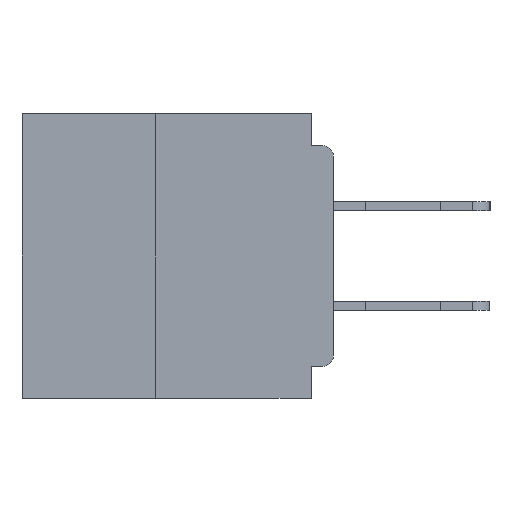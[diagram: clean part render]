
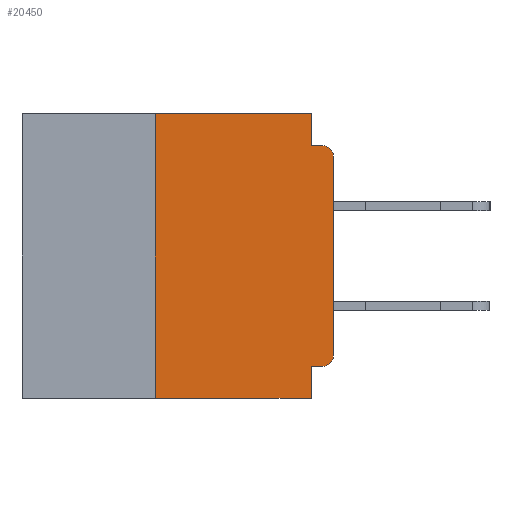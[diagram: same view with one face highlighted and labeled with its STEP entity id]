
A CAD part, left-side view. The second image highlights one B-rep face of the part: STEP entity #20450.
In plain terms, the highlighted planar face has unit normal (-1, 0, 0).
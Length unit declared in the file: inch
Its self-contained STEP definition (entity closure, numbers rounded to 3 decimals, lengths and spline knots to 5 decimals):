
#257 = EDGE_CURVE ( 'NONE', #21240, #16895, #29315, .T. ) ;
#332 = DIRECTION ( 'NONE',  ( -1., 0., 0. ) ) ;
#970 = CARTESIAN_POINT ( 'NONE',  ( 0., 0.015, -0.045 ) ) ;
#2657 = CARTESIAN_POINT ( 'NONE',  ( 0., 0.031, -0.045 ) ) ;
#2913 = LINE ( 'NONE', #9096, #38923 ) ;
#4142 = CARTESIAN_POINT ( 'NONE',  ( 0., 0., -0.34 ) ) ;
#5055 = VECTOR ( 'NONE', #23852, 39.37008 ) ;
#5239 = VERTEX_POINT ( 'NONE', #36201 ) ;
#6956 = VERTEX_POINT ( 'NONE', #32153 ) ;
#8666 = VERTEX_POINT ( 'NONE', #28612 ) ;
#9096 = CARTESIAN_POINT ( 'NONE',  ( 0., 0., 0. ) ) ;
#9192 = LINE ( 'NONE', #13168, #24970 ) ;
#9585 = VECTOR ( 'NONE', #23158, 39.37008 ) ;
#10369 = ORIENTED_EDGE ( 'NONE', *, *, #34134, .T. ) ;
#10654 = DIRECTION ( 'NONE',  ( 0., 0., -1. ) ) ;
#10909 = EDGE_CURVE ( 'NONE', #5239, #39149, #43585, .T. ) ;
#11137 = ORIENTED_EDGE ( 'NONE', *, *, #34809, .T. ) ;
#11266 = VERTEX_POINT ( 'NONE', #11587 ) ;
#11587 = CARTESIAN_POINT ( 'NONE',  ( 0., 0.25, -0.4 ) ) ;
#12026 = AXIS2_PLACEMENT_3D ( 'NONE', #34655, #13116, #38203 ) ;
#13116 = DIRECTION ( 'NONE',  ( -1., 0., 0. ) ) ;
#13168 = CARTESIAN_POINT ( 'NONE',  ( 0., 0.437, -0.4 ) ) ;
#13255 = ORIENTED_EDGE ( 'NONE', *, *, #10909, .F. ) ;
#13283 = ORIENTED_EDGE ( 'NONE', *, *, #257, .F. ) ;
#13321 = EDGE_CURVE ( 'NONE', #11266, #39149, #9192, .T. ) ;
#14574 = EDGE_CURVE ( 'NONE', #16895, #30800, #29369, .T. ) ;
#15464 = PLANE ( 'NONE',  #26780 ) ;
#16793 = EDGE_CURVE ( 'NONE', #6956, #5239, #33820, .T. ) ;
#16895 = VERTEX_POINT ( 'NONE', #2657 ) ;
#18525 = DIRECTION ( 'NONE',  ( 0., -1., 0. ) ) ;
#18948 = CARTESIAN_POINT ( 'NONE',  ( 0., 0.031, -0.4 ) ) ;
#19184 = LINE ( 'NONE', #37280, #9585 ) ;
#20450 = ADVANCED_FACE ( 'NONE', ( #27389 ), #15464, .F. ) ;
#20467 = DIRECTION ( 'NONE',  ( 0., 0., -1. ) ) ;
#21240 = VERTEX_POINT ( 'NONE', #41824 ) ;
#22002 = CARTESIAN_POINT ( 'NONE',  ( 0., 0.015, -0.06 ) ) ;
#22453 = DIRECTION ( 'NONE',  ( 0., 0., 1. ) ) ;
#22488 = CIRCLE ( 'NONE', #12026, 0.015 ) ;
#22690 = DIRECTION ( 'NONE',  ( 0., 0., -1. ) ) ;
#23158 = DIRECTION ( 'NONE',  ( 0., 0., 1. ) ) ;
#23670 = EDGE_CURVE ( 'NONE', #6956, #42886, #22488, .T. ) ;
#23852 = DIRECTION ( 'NONE',  ( 0., 1., 0. ) ) ;
#24042 = DIRECTION ( 'NONE',  ( 0., -1., 0. ) ) ;
#24398 = ORIENTED_EDGE ( 'NONE', *, *, #16793, .F. ) ;
#24970 = VECTOR ( 'NONE', #24042, 39.37008 ) ;
#24983 = ORIENTED_EDGE ( 'NONE', *, *, #13321, .T. ) ;
#25650 = DIRECTION ( 'NONE',  ( 0., 0., -1. ) ) ;
#26780 = AXIS2_PLACEMENT_3D ( 'NONE', #40483, #44033, #22690 ) ;
#27389 = FACE_OUTER_BOUND ( 'NONE', #42995, .T. ) ;
#28597 = ORIENTED_EDGE ( 'NONE', *, *, #14574, .F. ) ;
#28612 = CARTESIAN_POINT ( 'NONE',  ( 0., 0., -0.06 ) ) ;
#29315 = LINE ( 'NONE', #43407, #37644 ) ;
#29369 = LINE ( 'NONE', #38201, #44864 ) ;
#30227 = EDGE_CURVE ( 'NONE', #11266, #41132, #19184, .T. ) ;
#30800 = VERTEX_POINT ( 'NONE', #970 ) ;
#31580 = VECTOR ( 'NONE', #18525, 39.37008 ) ;
#32153 = CARTESIAN_POINT ( 'NONE',  ( 0., 0.015, -0.355 ) ) ;
#33820 = LINE ( 'NONE', #41613, #5055 ) ;
#34134 = EDGE_CURVE ( 'NONE', #42886, #8666, #2913, .T. ) ;
#34188 = VECTOR ( 'NONE', #20467, 39.37008 ) ;
#34655 = CARTESIAN_POINT ( 'NONE',  ( 0., 0.015, -0.34 ) ) ;
#34809 = EDGE_CURVE ( 'NONE', #8666, #30800, #37214, .T. ) ;
#36201 = CARTESIAN_POINT ( 'NONE',  ( 0., 0.031, -0.355 ) ) ;
#37214 = CIRCLE ( 'NONE', #44979, 0.015 ) ;
#37280 = CARTESIAN_POINT ( 'NONE',  ( 0., 0.25, -0.4 ) ) ;
#37644 = VECTOR ( 'NONE', #10654, 39.37008 ) ;
#38110 = ORIENTED_EDGE ( 'NONE', *, *, #44725, .F. ) ;
#38201 = CARTESIAN_POINT ( 'NONE',  ( 0., 0., -0.045 ) ) ;
#38203 = DIRECTION ( 'NONE',  ( 0., 0., -1. ) ) ;
#38281 = CARTESIAN_POINT ( 'NONE',  ( 0., 0.25, 0. ) ) ;
#38361 = DIRECTION ( 'NONE',  ( 0., -1., 0. ) ) ;
#38534 = ORIENTED_EDGE ( 'NONE', *, *, #30227, .F. ) ;
#38923 = VECTOR ( 'NONE', #22453, 39.37008 ) ;
#39149 = VERTEX_POINT ( 'NONE', #18948 ) ;
#39895 = LINE ( 'NONE', #43497, #31580 ) ;
#40483 = CARTESIAN_POINT ( 'NONE',  ( 0., 0.437, 0. ) ) ;
#41132 = VERTEX_POINT ( 'NONE', #38281 ) ;
#41613 = CARTESIAN_POINT ( 'NONE',  ( 0., 0., -0.355 ) ) ;
#41824 = CARTESIAN_POINT ( 'NONE',  ( 0., 0.031, 0. ) ) ;
#41851 = CARTESIAN_POINT ( 'NONE',  ( 0., 0.031, -0.4 ) ) ;
#42191 = ORIENTED_EDGE ( 'NONE', *, *, #23670, .T. ) ;
#42886 = VERTEX_POINT ( 'NONE', #4142 ) ;
#42995 = EDGE_LOOP ( 'NONE', ( #10369, #11137, #28597, #13283, #38110, #38534, #24983, #13255, #24398, #42191 ) ) ;
#43407 = CARTESIAN_POINT ( 'NONE',  ( 0., 0.031, 0. ) ) ;
#43497 = CARTESIAN_POINT ( 'NONE',  ( 0., 0.437, 0. ) ) ;
#43585 = LINE ( 'NONE', #41851, #34188 ) ;
#44033 = DIRECTION ( 'NONE',  ( 1., 0., 0. ) ) ;
#44725 = EDGE_CURVE ( 'NONE', #41132, #21240, #39895, .T. ) ;
#44864 = VECTOR ( 'NONE', #38361, 39.37008 ) ;
#44979 = AXIS2_PLACEMENT_3D ( 'NONE', #22002, #332, #25650 ) ;
